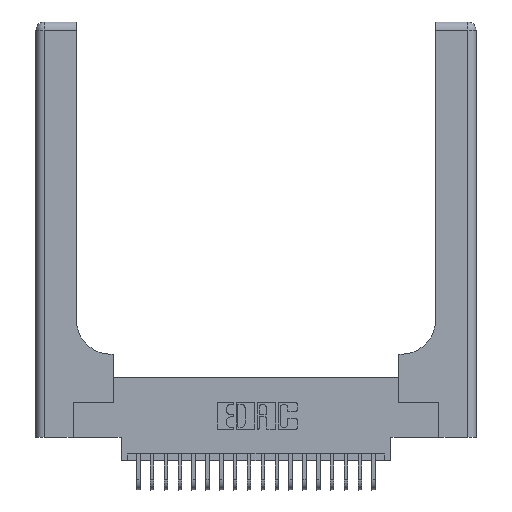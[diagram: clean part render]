
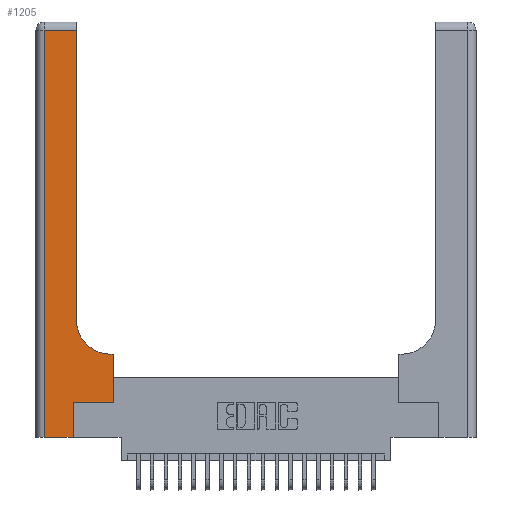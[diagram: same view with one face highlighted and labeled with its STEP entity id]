
A CAD part, top view. The second image highlights one B-rep face of the part: STEP entity #1205.
In plain terms, the highlighted planar face has unit normal (0, 0, 1).
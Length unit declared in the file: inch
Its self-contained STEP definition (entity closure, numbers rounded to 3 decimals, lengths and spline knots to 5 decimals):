
#473 = EDGE_CURVE ( 'NONE', #14555, #23076, #13374, .T. ) ;
#659 = VERTEX_POINT ( 'NONE', #19689 ) ;
#722 = DIRECTION ( 'NONE',  ( 0., 1., 0. ) ) ;
#1089 = CARTESIAN_POINT ( 'NONE',  ( 0.06, 2.94, 0.37 ) ) ;
#1205 = ADVANCED_FACE ( 'NONE', ( #9251 ), #2271, .F. ) ;
#1486 = EDGE_CURVE ( 'NONE', #15783, #14555, #3858, .T. ) ;
#2025 = CARTESIAN_POINT ( 'NONE',  ( 0.269, 0.25, 0.37 ) ) ;
#2100 = DIRECTION ( 'NONE',  ( -1., 0., 0. ) ) ;
#2151 = DIRECTION ( 'NONE',  ( 0., 0., -1. ) ) ;
#2194 = VERTEX_POINT ( 'NONE', #20812 ) ;
#2271 = PLANE ( 'NONE',  #9309 ) ;
#2421 = CARTESIAN_POINT ( 'NONE',  ( 0., 3., 0.37 ) ) ;
#2575 = CARTESIAN_POINT ( 'NONE',  ( 0.2915, 3., 0.37 ) ) ;
#3085 = CARTESIAN_POINT ( 'NONE',  ( 0., 0., 0.37 ) ) ;
#3283 = VECTOR ( 'NONE', #11038, 39.37008 ) ;
#3364 = DIRECTION ( 'NONE',  ( 0., -1., 0. ) ) ;
#3708 = DIRECTION ( 'NONE',  ( -1., 0., 0. ) ) ;
#3858 = LINE ( 'NONE', #9301, #13327 ) ;
#3947 = DIRECTION ( 'NONE',  ( 0., 0., -1. ) ) ;
#4547 = EDGE_CURVE ( 'NONE', #13329, #19258, #13365, .T. ) ;
#4724 = CARTESIAN_POINT ( 'NONE',  ( 0.5585, 0.25, 0.37 ) ) ;
#5218 = DIRECTION ( 'NONE',  ( 1., 0., 0. ) ) ;
#5248 = EDGE_LOOP ( 'NONE', ( #21388, #7434, #22594, #10412, #16650, #15167, #23676, #18542, #10826 ) ) ;
#5409 = EDGE_CURVE ( 'NONE', #23076, #13329, #23228, .T. ) ;
#5591 = CARTESIAN_POINT ( 'NONE',  ( 0.2915, 0.6, 0.37 ) ) ;
#6989 = CARTESIAN_POINT ( 'NONE',  ( 0.269, 0., 0.37 ) ) ;
#7434 = ORIENTED_EDGE ( 'NONE', *, *, #23173, .T. ) ;
#8173 = CIRCLE ( 'NONE', #9595, 0.25 ) ;
#8579 = DIRECTION ( 'NONE',  ( 0., 1., 0. ) ) ;
#9251 = FACE_OUTER_BOUND ( 'NONE', #5248, .T. ) ;
#9301 = CARTESIAN_POINT ( 'NONE',  ( 0.269, 0., 0.37 ) ) ;
#9309 = AXIS2_PLACEMENT_3D ( 'NONE', #2421, #2151, #2100 ) ;
#9595 = AXIS2_PLACEMENT_3D ( 'NONE', #15281, #3947, #17174 ) ;
#10118 = EDGE_CURVE ( 'NONE', #2194, #15783, #20708, .T. ) ;
#10412 = ORIENTED_EDGE ( 'NONE', *, *, #10118, .T. ) ;
#10826 = ORIENTED_EDGE ( 'NONE', *, *, #15143, .T. ) ;
#11038 = DIRECTION ( 'NONE',  ( -1., 0., 0. ) ) ;
#11904 = VERTEX_POINT ( 'NONE', #1089 ) ;
#11927 = VERTEX_POINT ( 'NONE', #12460 ) ;
#12460 = CARTESIAN_POINT ( 'NONE',  ( 0.2915, 2.94, 0.37 ) ) ;
#12465 = EDGE_CURVE ( 'NONE', #659, #11927, #23748, .T. ) ;
#12749 = VECTOR ( 'NONE', #8579, 39.37008 ) ;
#12808 = CARTESIAN_POINT ( 'NONE',  ( 0.06, 3., 0.37 ) ) ;
#12820 = CARTESIAN_POINT ( 'NONE',  ( 0., 2.94, 0.37 ) ) ;
#13327 = VECTOR ( 'NONE', #22365, 39.37008 ) ;
#13329 = VERTEX_POINT ( 'NONE', #24048 ) ;
#13365 = LINE ( 'NONE', #5591, #13974 ) ;
#13374 = LINE ( 'NONE', #2025, #18982 ) ;
#13974 = VECTOR ( 'NONE', #3708, 39.37008 ) ;
#14555 = VERTEX_POINT ( 'NONE', #15150 ) ;
#15143 = EDGE_CURVE ( 'NONE', #19258, #659, #8173, .T. ) ;
#15150 = CARTESIAN_POINT ( 'NONE',  ( 0.269, 0.25, 0.37 ) ) ;
#15167 = ORIENTED_EDGE ( 'NONE', *, *, #473, .T. ) ;
#15206 = LINE ( 'NONE', #12808, #19029 ) ;
#15281 = CARTESIAN_POINT ( 'NONE',  ( 0.5415, 0.85, 0.37 ) ) ;
#15733 = VECTOR ( 'NONE', #21918, 39.37008 ) ;
#15783 = VERTEX_POINT ( 'NONE', #6989 ) ;
#16650 = ORIENTED_EDGE ( 'NONE', *, *, #1486, .T. ) ;
#17170 = LINE ( 'NONE', #12820, #3283 ) ;
#17174 = DIRECTION ( 'NONE',  ( 1., 0., 0. ) ) ;
#18392 = CARTESIAN_POINT ( 'NONE',  ( 0.5415, 0.6, 0.37 ) ) ;
#18542 = ORIENTED_EDGE ( 'NONE', *, *, #4547, .T. ) ;
#18870 = VECTOR ( 'NONE', #722, 39.37008 ) ;
#18982 = VECTOR ( 'NONE', #5218, 39.37008 ) ;
#19029 = VECTOR ( 'NONE', #3364, 39.37008 ) ;
#19258 = VERTEX_POINT ( 'NONE', #18392 ) ;
#19689 = CARTESIAN_POINT ( 'NONE',  ( 0.2915, 0.85, 0.37 ) ) ;
#20437 = EDGE_CURVE ( 'NONE', #11904, #2194, #15206, .T. ) ;
#20708 = LINE ( 'NONE', #3085, #15733 ) ;
#20812 = CARTESIAN_POINT ( 'NONE',  ( 0.06, 0., 0.37 ) ) ;
#21388 = ORIENTED_EDGE ( 'NONE', *, *, #12465, .T. ) ;
#21918 = DIRECTION ( 'NONE',  ( 1., 0., 0. ) ) ;
#22365 = DIRECTION ( 'NONE',  ( 0., 1., 0. ) ) ;
#22594 = ORIENTED_EDGE ( 'NONE', *, *, #20437, .T. ) ;
#23076 = VERTEX_POINT ( 'NONE', #23405 ) ;
#23173 = EDGE_CURVE ( 'NONE', #11927, #11904, #17170, .T. ) ;
#23228 = LINE ( 'NONE', #4724, #12749 ) ;
#23405 = CARTESIAN_POINT ( 'NONE',  ( 0.5585, 0.25, 0.37 ) ) ;
#23676 = ORIENTED_EDGE ( 'NONE', *, *, #5409, .T. ) ;
#23748 = LINE ( 'NONE', #2575, #18870 ) ;
#24048 = CARTESIAN_POINT ( 'NONE',  ( 0.5585, 0.6, 0.37 ) ) ;
